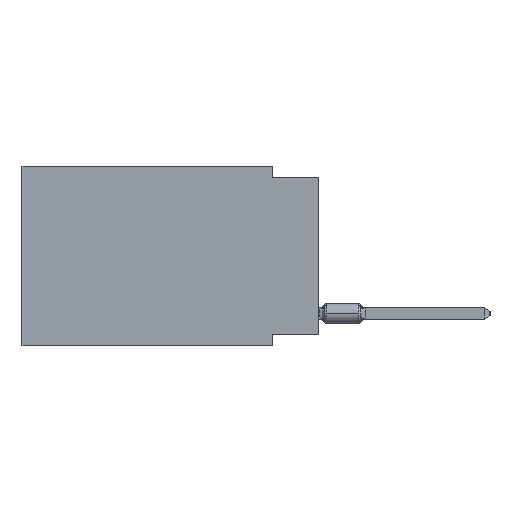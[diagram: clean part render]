
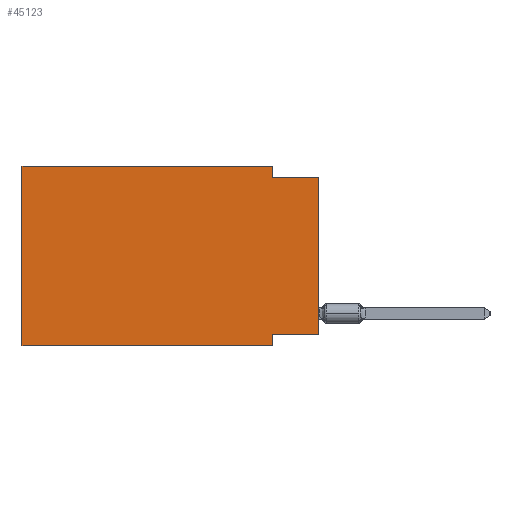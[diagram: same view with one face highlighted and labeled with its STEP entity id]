
A CAD part, left-side view. The second image highlights one B-rep face of the part: STEP entity #45123.
In plain terms, the highlighted planar face has unit normal (-1, 0, 0).
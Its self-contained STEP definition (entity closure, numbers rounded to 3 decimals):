
#598 = CARTESIAN_POINT ( 'NONE',  ( 0., 2.54, -9.271 ) ) ;
#1089 = LINE ( 'NONE', #34386, #38220 ) ;
#1112 = CARTESIAN_POINT ( 'NONE',  ( 0., 16.383, -9.906 ) ) ;
#3623 = VECTOR ( 'NONE', #37707, 1000. ) ;
#4406 = CARTESIAN_POINT ( 'NONE',  ( 0., 16.383, 0. ) ) ;
#4512 = EDGE_CURVE ( 'NONE', #49786, #38095, #52263, .T. ) ;
#5209 = DIRECTION ( 'NONE',  ( 0., -1., 0. ) ) ;
#6047 = CARTESIAN_POINT ( 'NONE',  ( 0., 2.54, 0. ) ) ;
#6057 = EDGE_CURVE ( 'NONE', #13332, #49786, #51542, .T. ) ;
#9514 = CARTESIAN_POINT ( 'NONE',  ( 0., 0., -0.635 ) ) ;
#9864 = VECTOR ( 'NONE', #5209, 1000. ) ;
#9957 = DIRECTION ( 'NONE',  ( 0., 0., -1. ) ) ;
#10851 = LINE ( 'NONE', #26441, #32694 ) ;
#12838 = CARTESIAN_POINT ( 'NONE',  ( 0., 2.54, -9.906 ) ) ;
#13246 = CARTESIAN_POINT ( 'NONE',  ( 0., 2.54, -9.906 ) ) ;
#13332 = VERTEX_POINT ( 'NONE', #43225 ) ;
#14630 = EDGE_CURVE ( 'NONE', #24988, #28812, #15999, .T. ) ;
#15999 = LINE ( 'NONE', #4406, #3623 ) ;
#16897 = ORIENTED_EDGE ( 'NONE', *, *, #16967, .F. ) ;
#16967 = EDGE_CURVE ( 'NONE', #41781, #33104, #50551, .T. ) ;
#21108 = EDGE_CURVE ( 'NONE', #24988, #33104, #51228, .T. ) ;
#21996 = DIRECTION ( 'NONE',  ( 0., 0., -1. ) ) ;
#22364 = VECTOR ( 'NONE', #9957, 1000. ) ;
#22400 = DIRECTION ( 'NONE',  ( 0., 1., 0. ) ) ;
#23420 = CARTESIAN_POINT ( 'NONE',  ( 0., 16.383, 0. ) ) ;
#23801 = ORIENTED_EDGE ( 'NONE', *, *, #28417, .F. ) ;
#24988 = VERTEX_POINT ( 'NONE', #38551 ) ;
#25246 = CARTESIAN_POINT ( 'NONE',  ( 0., 2.54, -0.635 ) ) ;
#25548 = CARTESIAN_POINT ( 'NONE',  ( 0., 16.383, 0. ) ) ;
#26080 = EDGE_CURVE ( 'NONE', #28812, #13332, #10851, .T. ) ;
#26358 = FACE_OUTER_BOUND ( 'NONE', #53253, .T. ) ;
#26441 = CARTESIAN_POINT ( 'NONE',  ( 0., 16.383, 0. ) ) ;
#28417 = EDGE_CURVE ( 'NONE', #42801, #41781, #1089, .T. ) ;
#28571 = ORIENTED_EDGE ( 'NONE', *, *, #21108, .T. ) ;
#28750 = VECTOR ( 'NONE', #39255, 1000. ) ;
#28812 = VERTEX_POINT ( 'NONE', #23420 ) ;
#30551 = VECTOR ( 'NONE', #50728, 1000. ) ;
#30773 = ORIENTED_EDGE ( 'NONE', *, *, #26080, .F. ) ;
#32152 = AXIS2_PLACEMENT_3D ( 'NONE', #25548, #51059, #21996 ) ;
#32694 = VECTOR ( 'NONE', #47621, 1000. ) ;
#33104 = VERTEX_POINT ( 'NONE', #12838 ) ;
#34386 = CARTESIAN_POINT ( 'NONE',  ( 0., 0., -9.271 ) ) ;
#35123 = EDGE_CURVE ( 'NONE', #42801, #38095, #48346, .T. ) ;
#35322 = CARTESIAN_POINT ( 'NONE',  ( 0., 0., 0. ) ) ;
#37707 = DIRECTION ( 'NONE',  ( 0., 0., 1. ) ) ;
#37954 = ORIENTED_EDGE ( 'NONE', *, *, #35123, .T. ) ;
#38095 = VERTEX_POINT ( 'NONE', #49740 ) ;
#38220 = VECTOR ( 'NONE', #22400, 1000. ) ;
#38551 = CARTESIAN_POINT ( 'NONE',  ( 0., 16.383, -9.906 ) ) ;
#39255 = DIRECTION ( 'NONE',  ( 0., -1., 0. ) ) ;
#39317 = ORIENTED_EDGE ( 'NONE', *, *, #14630, .F. ) ;
#40013 = CARTESIAN_POINT ( 'NONE',  ( 0., 0., -9.271 ) ) ;
#40286 = ORIENTED_EDGE ( 'NONE', *, *, #6057, .F. ) ;
#41781 = VERTEX_POINT ( 'NONE', #598 ) ;
#42801 = VERTEX_POINT ( 'NONE', #40013 ) ;
#43225 = CARTESIAN_POINT ( 'NONE',  ( 0., 2.54, 0. ) ) ;
#44553 = DIRECTION ( 'NONE',  ( 0., 0., 1. ) ) ;
#45123 = ADVANCED_FACE ( 'NONE', ( #26358 ), #50534, .F. ) ;
#47438 = ORIENTED_EDGE ( 'NONE', *, *, #4512, .F. ) ;
#47621 = DIRECTION ( 'NONE',  ( 0., -1., 0. ) ) ;
#48346 = LINE ( 'NONE', #35322, #51803 ) ;
#49740 = CARTESIAN_POINT ( 'NONE',  ( 0., 0., -0.635 ) ) ;
#49786 = VERTEX_POINT ( 'NONE', #25246 ) ;
#50534 = PLANE ( 'NONE',  #32152 ) ;
#50551 = LINE ( 'NONE', #13246, #22364 ) ;
#50728 = DIRECTION ( 'NONE',  ( 0., 0., -1. ) ) ;
#51059 = DIRECTION ( 'NONE',  ( 1., 0., 0. ) ) ;
#51228 = LINE ( 'NONE', #1112, #9864 ) ;
#51542 = LINE ( 'NONE', #6047, #30551 ) ;
#51803 = VECTOR ( 'NONE', #44553, 1000. ) ;
#52263 = LINE ( 'NONE', #9514, #28750 ) ;
#53253 = EDGE_LOOP ( 'NONE', ( #37954, #47438, #40286, #30773, #39317, #28571, #16897, #23801 ) ) ;
